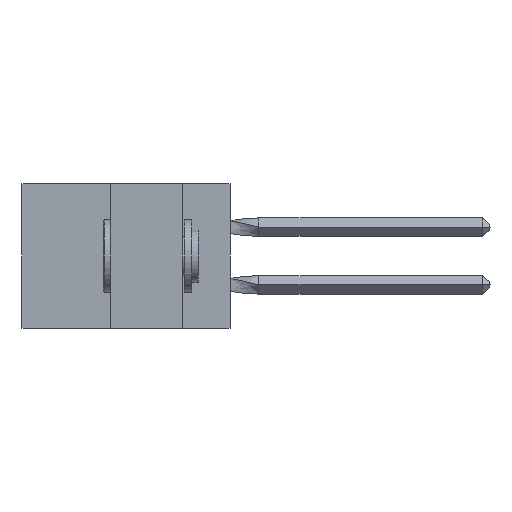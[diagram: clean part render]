
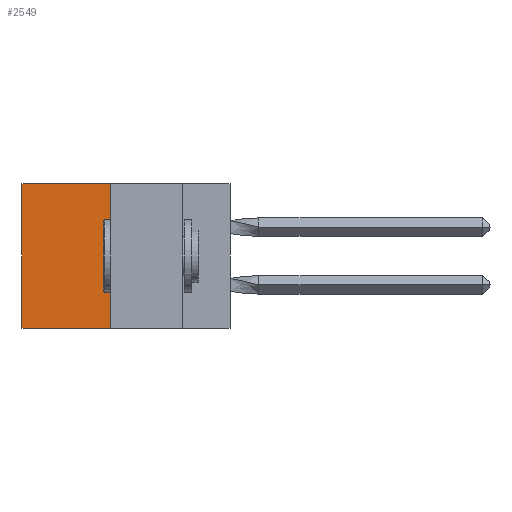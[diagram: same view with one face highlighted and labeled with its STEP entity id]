
A CAD part, left-side view. The second image highlights one B-rep face of the part: STEP entity #2549.
In plain terms, the highlighted planar face has unit normal (-1, 0, 0).
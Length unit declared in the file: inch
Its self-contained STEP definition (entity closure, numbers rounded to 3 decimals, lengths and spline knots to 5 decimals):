
#1513 = PLANE ( 'NONE',  #7498 ) ;
#1678 = DIRECTION ( 'NONE',  ( 1., 0., 0. ) ) ;
#2329 = ORIENTED_EDGE ( 'NONE', *, *, #14795, .F. ) ;
#2522 = EDGE_LOOP ( 'NONE', ( #12054, #7713, #2329, #11135 ) ) ;
#2549 = ADVANCED_FACE ( 'NONE', ( #14573 ), #1513, .F. ) ;
#2702 = CARTESIAN_POINT ( 'NONE',  ( 0.305, 0.72, 0. ) ) ;
#2741 = CARTESIAN_POINT ( 'NONE',  ( 0.305, 0.413, 0. ) ) ;
#3264 = CARTESIAN_POINT ( 'NONE',  ( 0.305, 0.72, -0.5 ) ) ;
#3705 = EDGE_CURVE ( 'NONE', #9474, #8975, #15312, .T. ) ;
#4646 = VERTEX_POINT ( 'NONE', #2702 ) ;
#4905 = LINE ( 'NONE', #2741, #11542 ) ;
#5140 = LINE ( 'NONE', #14291, #8006 ) ;
#5191 = EDGE_CURVE ( 'NONE', #10207, #4646, #4905, .T. ) ;
#6578 = DIRECTION ( 'NONE',  ( 0., 1., 0. ) ) ;
#6798 = CARTESIAN_POINT ( 'NONE',  ( 0.305, 0.413, -0.5 ) ) ;
#7498 = AXIS2_PLACEMENT_3D ( 'NONE', #11202, #1678, #8805 ) ;
#7713 = ORIENTED_EDGE ( 'NONE', *, *, #3705, .F. ) ;
#7791 = CARTESIAN_POINT ( 'NONE',  ( 0.305, 0.72, -0.5 ) ) ;
#8006 = VECTOR ( 'NONE', #11986, 39.37008 ) ;
#8805 = DIRECTION ( 'NONE',  ( 0., 0., -1. ) ) ;
#8975 = VERTEX_POINT ( 'NONE', #7791 ) ;
#9036 = CARTESIAN_POINT ( 'NONE',  ( 0.305, 0.413, -0.5 ) ) ;
#9474 = VERTEX_POINT ( 'NONE', #9036 ) ;
#9846 = CARTESIAN_POINT ( 'NONE',  ( 0.305, 0.413, 0. ) ) ;
#10126 = EDGE_CURVE ( 'NONE', #4646, #8975, #11034, .T. ) ;
#10207 = VERTEX_POINT ( 'NONE', #9846 ) ;
#11034 = LINE ( 'NONE', #3264, #11777 ) ;
#11135 = ORIENTED_EDGE ( 'NONE', *, *, #5191, .T. ) ;
#11202 = CARTESIAN_POINT ( 'NONE',  ( 0.305, 0.413, -0.5 ) ) ;
#11542 = VECTOR ( 'NONE', #13565, 39.37008 ) ;
#11711 = DIRECTION ( 'NONE',  ( 0., 0., -1. ) ) ;
#11777 = VECTOR ( 'NONE', #11711, 39.37008 ) ;
#11986 = DIRECTION ( 'NONE',  ( 0., 0., -1. ) ) ;
#12054 = ORIENTED_EDGE ( 'NONE', *, *, #10126, .T. ) ;
#13259 = VECTOR ( 'NONE', #6578, 39.37008 ) ;
#13565 = DIRECTION ( 'NONE',  ( 0., 1., 0. ) ) ;
#14291 = CARTESIAN_POINT ( 'NONE',  ( 0.305, 0.413, -0.5 ) ) ;
#14573 = FACE_OUTER_BOUND ( 'NONE', #2522, .T. ) ;
#14795 = EDGE_CURVE ( 'NONE', #10207, #9474, #5140, .T. ) ;
#15312 = LINE ( 'NONE', #6798, #13259 ) ;
